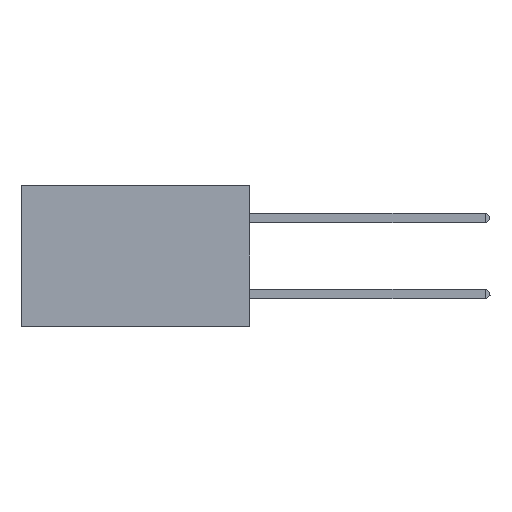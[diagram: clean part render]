
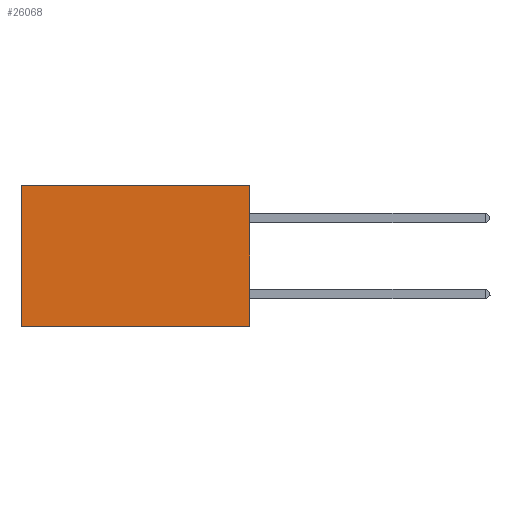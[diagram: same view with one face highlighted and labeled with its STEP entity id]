
A CAD part, left-side view. The second image highlights one B-rep face of the part: STEP entity #26068.
In plain terms, the highlighted planar face has unit normal (-1, 0, 0).
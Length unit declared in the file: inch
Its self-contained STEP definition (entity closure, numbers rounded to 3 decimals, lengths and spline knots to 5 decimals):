
#263 = CARTESIAN_POINT ( 'NONE',  ( 0.2875, 0., -0.37 ) ) ;
#884 = VERTEX_POINT ( 'NONE', #17567 ) ;
#2868 = VERTEX_POINT ( 'NONE', #15436 ) ;
#3544 = DIRECTION ( 'NONE',  ( 0., 0., -1. ) ) ;
#4119 = PLANE ( 'NONE',  #20937 ) ;
#4998 = LINE ( 'NONE', #10156, #13029 ) ;
#5691 = DIRECTION ( 'NONE',  ( 0., 0., -1. ) ) ;
#7071 = VECTOR ( 'NONE', #10927, 39.37008 ) ;
#9425 = VECTOR ( 'NONE', #34876, 39.37008 ) ;
#10050 = VERTEX_POINT ( 'NONE', #38653 ) ;
#10156 = CARTESIAN_POINT ( 'NONE',  ( 0.2875, 0.6, 0. ) ) ;
#10766 = LINE ( 'NONE', #23623, #18759 ) ;
#10927 = DIRECTION ( 'NONE',  ( 0., 1., 0. ) ) ;
#13029 = VECTOR ( 'NONE', #3544, 39.37008 ) ;
#14247 = LINE ( 'NONE', #31137, #9425 ) ;
#14533 = ORIENTED_EDGE ( 'NONE', *, *, #33907, .F. ) ;
#15436 = CARTESIAN_POINT ( 'NONE',  ( 0.2875, 0., 0. ) ) ;
#16795 = ORIENTED_EDGE ( 'NONE', *, *, #22292, .T. ) ;
#17567 = CARTESIAN_POINT ( 'NONE',  ( 0.2875, 0., -0.37 ) ) ;
#18287 = LINE ( 'NONE', #263, #7071 ) ;
#18371 = ORIENTED_EDGE ( 'NONE', *, *, #42806, .T. ) ;
#18483 = ORIENTED_EDGE ( 'NONE', *, *, #23307, .F. ) ;
#18759 = VECTOR ( 'NONE', #37118, 39.37008 ) ;
#19002 = CARTESIAN_POINT ( 'NONE',  ( 0.2875, 0., 0. ) ) ;
#20242 = VERTEX_POINT ( 'NONE', #37547 ) ;
#20937 = AXIS2_PLACEMENT_3D ( 'NONE', #19002, #32779, #5691 ) ;
#22292 = EDGE_CURVE ( 'NONE', #10050, #20242, #4998, .T. ) ;
#23307 = EDGE_CURVE ( 'NONE', #884, #20242, #18287, .T. ) ;
#23623 = CARTESIAN_POINT ( 'NONE',  ( 0.2875, 0., 0. ) ) ;
#26068 = ADVANCED_FACE ( 'NONE', ( #39026 ), #4119, .F. ) ;
#31137 = CARTESIAN_POINT ( 'NONE',  ( 0.2875, 0., 0. ) ) ;
#32779 = DIRECTION ( 'NONE',  ( 1., 0., 0. ) ) ;
#33907 = EDGE_CURVE ( 'NONE', #2868, #884, #10766, .T. ) ;
#34876 = DIRECTION ( 'NONE',  ( 0., 1., 0. ) ) ;
#37118 = DIRECTION ( 'NONE',  ( 0., 0., -1. ) ) ;
#37547 = CARTESIAN_POINT ( 'NONE',  ( 0.2875, 0.6, -0.37 ) ) ;
#37599 = EDGE_LOOP ( 'NONE', ( #16795, #18483, #14533, #18371 ) ) ;
#38653 = CARTESIAN_POINT ( 'NONE',  ( 0.2875, 0.6, 0. ) ) ;
#39026 = FACE_OUTER_BOUND ( 'NONE', #37599, .T. ) ;
#42806 = EDGE_CURVE ( 'NONE', #2868, #10050, #14247, .T. ) ;
